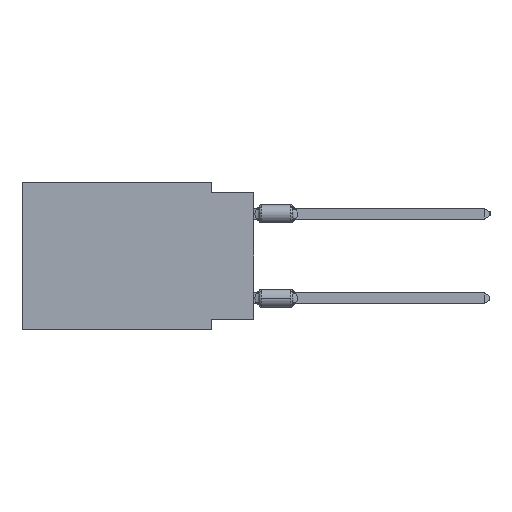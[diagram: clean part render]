
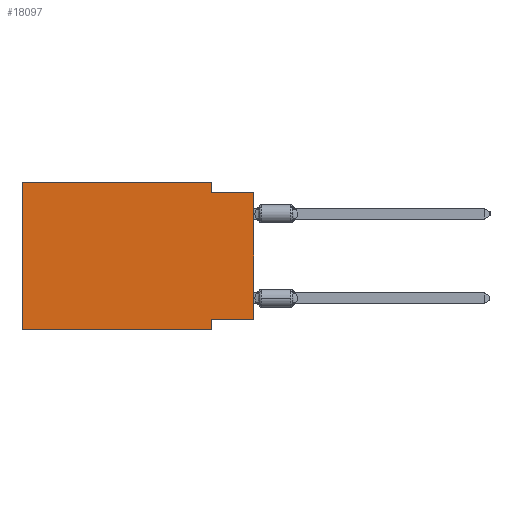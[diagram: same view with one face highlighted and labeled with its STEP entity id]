
A CAD part, left-side view. The second image highlights one B-rep face of the part: STEP entity #18097.
In plain terms, the highlighted planar face has unit normal (-1, 0, 0).
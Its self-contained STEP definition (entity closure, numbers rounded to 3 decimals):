
#1374 = DIRECTION ( 'NONE',  ( 0., -1., 0. ) ) ;
#2038 = VERTEX_POINT ( 'NONE', #18539 ) ;
#4364 = ORIENTED_EDGE ( 'NONE', *, *, #40391, .F. ) ;
#4514 = VECTOR ( 'NONE', #12956, 1000. ) ;
#4996 = ORIENTED_EDGE ( 'NONE', *, *, #20341, .F. ) ;
#5713 = VECTOR ( 'NONE', #32646, 1000. ) ;
#7227 = EDGE_CURVE ( 'NONE', #28563, #8420, #39569, .T. ) ;
#8420 = VERTEX_POINT ( 'NONE', #20644 ) ;
#9221 = EDGE_LOOP ( 'NONE', ( #30219, #4996, #4364, #40848, #42932, #26229, #21502, #12904 ) ) ;
#10385 = CARTESIAN_POINT ( 'NONE',  ( 0., 13.97, 0. ) ) ;
#10826 = VERTEX_POINT ( 'NONE', #19468 ) ;
#11116 = DIRECTION ( 'NONE',  ( 0., 0., -1. ) ) ;
#12904 = ORIENTED_EDGE ( 'NONE', *, *, #45934, .F. ) ;
#12956 = DIRECTION ( 'NONE',  ( 0., 0., -1. ) ) ;
#12973 = LINE ( 'NONE', #43039, #16590 ) ;
#13360 = CARTESIAN_POINT ( 'NONE',  ( 0., 0., -0.635 ) ) ;
#14224 = DIRECTION ( 'NONE',  ( 0., 1., 0. ) ) ;
#15087 = EDGE_CURVE ( 'NONE', #46158, #10826, #40495, .T. ) ;
#16590 = VECTOR ( 'NONE', #1374, 1000. ) ;
#16617 = CARTESIAN_POINT ( 'NONE',  ( 0., 13.97, 0. ) ) ;
#17882 = VECTOR ( 'NONE', #25100, 1000. ) ;
#17945 = EDGE_CURVE ( 'NONE', #32810, #28563, #29575, .T. ) ;
#18020 = LINE ( 'NONE', #24861, #30398 ) ;
#18097 = ADVANCED_FACE ( 'NONE', ( #19676 ), #35091, .F. ) ;
#18137 = LINE ( 'NONE', #13360, #27088 ) ;
#18539 = CARTESIAN_POINT ( 'NONE',  ( 0., 2.54, -0.635 ) ) ;
#19468 = CARTESIAN_POINT ( 'NONE',  ( 0., 2.54, -8.89 ) ) ;
#19676 = FACE_OUTER_BOUND ( 'NONE', #9221, .T. ) ;
#19946 = CARTESIAN_POINT ( 'NONE',  ( 0., 13.97, 0. ) ) ;
#20341 = EDGE_CURVE ( 'NONE', #2038, #25491, #18137, .T. ) ;
#20644 = CARTESIAN_POINT ( 'NONE',  ( 0., 2.54, 0. ) ) ;
#21502 = ORIENTED_EDGE ( 'NONE', *, *, #15087, .F. ) ;
#22619 = EDGE_CURVE ( 'NONE', #40516, #25491, #37162, .T. ) ;
#24861 = CARTESIAN_POINT ( 'NONE',  ( 0., 0., -8.255 ) ) ;
#25054 = CARTESIAN_POINT ( 'NONE',  ( 0., 0., 0. ) ) ;
#25100 = DIRECTION ( 'NONE',  ( 0., 0., -1. ) ) ;
#25491 = VERTEX_POINT ( 'NONE', #46505 ) ;
#25771 = DIRECTION ( 'NONE',  ( 0., 0., 1. ) ) ;
#26051 = CARTESIAN_POINT ( 'NONE',  ( 0., 0., -8.255 ) ) ;
#26210 = AXIS2_PLACEMENT_3D ( 'NONE', #19946, #35357, #11116 ) ;
#26229 = ORIENTED_EDGE ( 'NONE', *, *, #44696, .T. ) ;
#27088 = VECTOR ( 'NONE', #33556, 1000. ) ;
#28563 = VERTEX_POINT ( 'NONE', #16617 ) ;
#28908 = CARTESIAN_POINT ( 'NONE',  ( 0., 2.54, -8.89 ) ) ;
#29123 = LINE ( 'NONE', #32671, #4514 ) ;
#29575 = LINE ( 'NONE', #10385, #34293 ) ;
#30219 = ORIENTED_EDGE ( 'NONE', *, *, #22619, .T. ) ;
#30398 = VECTOR ( 'NONE', #14224, 1000. ) ;
#32646 = DIRECTION ( 'NONE',  ( 0., 0., 1. ) ) ;
#32671 = CARTESIAN_POINT ( 'NONE',  ( 0., 2.54, 0. ) ) ;
#32810 = VERTEX_POINT ( 'NONE', #46273 ) ;
#33556 = DIRECTION ( 'NONE',  ( 0., -1., 0. ) ) ;
#34158 = CARTESIAN_POINT ( 'NONE',  ( 0., 2.54, -8.255 ) ) ;
#34293 = VECTOR ( 'NONE', #25771, 1000. ) ;
#35091 = PLANE ( 'NONE',  #26210 ) ;
#35357 = DIRECTION ( 'NONE',  ( 1., 0., 0. ) ) ;
#37162 = LINE ( 'NONE', #25054, #5713 ) ;
#39569 = LINE ( 'NONE', #47407, #45181 ) ;
#40391 = EDGE_CURVE ( 'NONE', #8420, #2038, #29123, .T. ) ;
#40495 = LINE ( 'NONE', #28908, #17882 ) ;
#40516 = VERTEX_POINT ( 'NONE', #26051 ) ;
#40848 = ORIENTED_EDGE ( 'NONE', *, *, #7227, .F. ) ;
#42932 = ORIENTED_EDGE ( 'NONE', *, *, #17945, .F. ) ;
#43039 = CARTESIAN_POINT ( 'NONE',  ( 0., 13.97, -8.89 ) ) ;
#44696 = EDGE_CURVE ( 'NONE', #32810, #10826, #12973, .T. ) ;
#45181 = VECTOR ( 'NONE', #47154, 1000. ) ;
#45934 = EDGE_CURVE ( 'NONE', #40516, #46158, #18020, .T. ) ;
#46158 = VERTEX_POINT ( 'NONE', #34158 ) ;
#46273 = CARTESIAN_POINT ( 'NONE',  ( 0., 13.97, -8.89 ) ) ;
#46505 = CARTESIAN_POINT ( 'NONE',  ( 0., 0., -0.635 ) ) ;
#47154 = DIRECTION ( 'NONE',  ( 0., -1., 0. ) ) ;
#47407 = CARTESIAN_POINT ( 'NONE',  ( 0., 13.97, 0. ) ) ;
